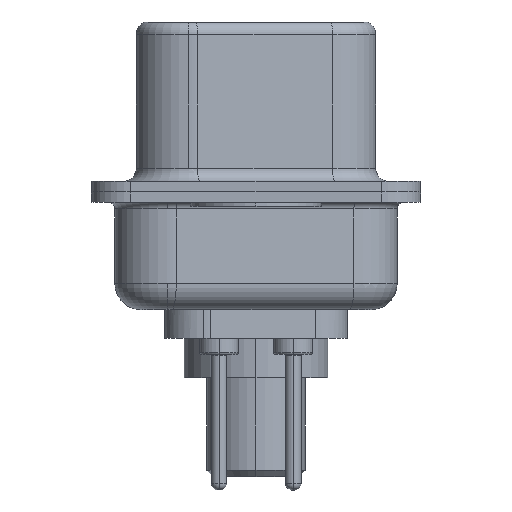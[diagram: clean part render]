
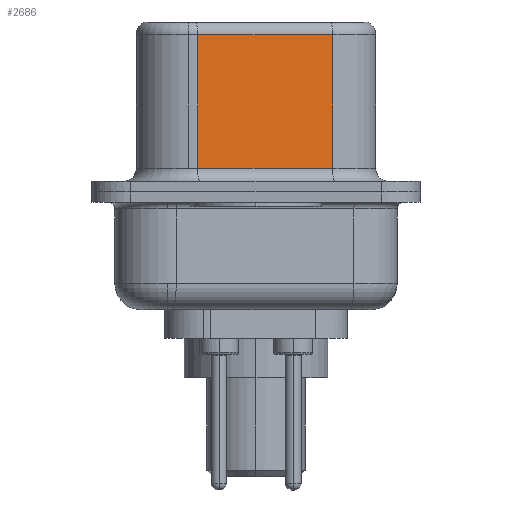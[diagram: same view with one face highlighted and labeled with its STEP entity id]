
A CAD part, left-side view. The second image highlights one B-rep face of the part: STEP entity #2686.
In plain terms, the highlighted planar face has unit normal (-0.985, -0.174, 0).
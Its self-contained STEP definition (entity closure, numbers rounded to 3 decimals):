
#196 = ORIENTED_EDGE ( 'NONE', *, *, #2378, .T. ) ;
#406 = AXIS2_PLACEMENT_3D ( 'NONE', #6512, #8771, #14631 ) ;
#682 = CARTESIAN_POINT ( 'NONE',  ( 4.565, -2.927, 6.52 ) ) ;
#2378 = EDGE_CURVE ( 'NONE', #8710, #3685, #7157, .T. ) ;
#2686 = ADVANCED_FACE ( 'NONE', ( #12148 ), #6078, .F. ) ;
#3644 = VECTOR ( 'NONE', #11291, 1000. ) ;
#3685 = VERTEX_POINT ( 'NONE', #7991 ) ;
#4021 = VECTOR ( 'NONE', #14158, 1000. ) ;
#4228 = VERTEX_POINT ( 'NONE', #9756 ) ;
#5491 = CARTESIAN_POINT ( 'NONE',  ( 4.565, -2.927, 0.9 ) ) ;
#6033 = LINE ( 'NONE', #5491, #13088 ) ;
#6078 = PLANE ( 'NONE',  #406 ) ;
#6512 = CARTESIAN_POINT ( 'NONE',  ( 4.565, -2.927, 6.52 ) ) ;
#7157 = LINE ( 'NONE', #9382, #4021 ) ;
#7173 = LINE ( 'NONE', #682, #3644 ) ;
#7906 = ORIENTED_EDGE ( 'NONE', *, *, #10077, .T. ) ;
#7991 = CARTESIAN_POINT ( 'NONE',  ( 3.655, 2.233, 0.9 ) ) ;
#8673 = CARTESIAN_POINT ( 'NONE',  ( 3.655, 2.233, 6.02 ) ) ;
#8710 = VERTEX_POINT ( 'NONE', #8673 ) ;
#8771 = DIRECTION ( 'NONE',  ( 0.985, 0.174, 0. ) ) ;
#8852 = DIRECTION ( 'NONE',  ( -0.174, 0.985, 0. ) ) ;
#9040 = DIRECTION ( 'NONE',  ( 0.174, -0.985, 0. ) ) ;
#9216 = ORIENTED_EDGE ( 'NONE', *, *, #13995, .F. ) ;
#9382 = CARTESIAN_POINT ( 'NONE',  ( 3.655, 2.233, 6.52 ) ) ;
#9598 = EDGE_LOOP ( 'NONE', ( #9216, #7906, #196, #11988 ) ) ;
#9693 = VECTOR ( 'NONE', #8852, 1000. ) ;
#9756 = CARTESIAN_POINT ( 'NONE',  ( 4.565, -2.927, 0.9 ) ) ;
#10077 = EDGE_CURVE ( 'NONE', #12723, #8710, #12809, .T. ) ;
#11291 = DIRECTION ( 'NONE',  ( 0., 0., -1. ) ) ;
#11988 = ORIENTED_EDGE ( 'NONE', *, *, #14100, .T. ) ;
#12148 = FACE_OUTER_BOUND ( 'NONE', #9598, .T. ) ;
#12334 = CARTESIAN_POINT ( 'NONE',  ( 4.565, -2.927, 6.02 ) ) ;
#12723 = VERTEX_POINT ( 'NONE', #13815 ) ;
#12809 = LINE ( 'NONE', #12334, #9693 ) ;
#13088 = VECTOR ( 'NONE', #9040, 1000. ) ;
#13815 = CARTESIAN_POINT ( 'NONE',  ( 4.565, -2.927, 6.02 ) ) ;
#13995 = EDGE_CURVE ( 'NONE', #12723, #4228, #7173, .T. ) ;
#14100 = EDGE_CURVE ( 'NONE', #3685, #4228, #6033, .T. ) ;
#14158 = DIRECTION ( 'NONE',  ( 0., 0., -1. ) ) ;
#14631 = DIRECTION ( 'NONE',  ( -0.174, 0.985, 0. ) ) ;
